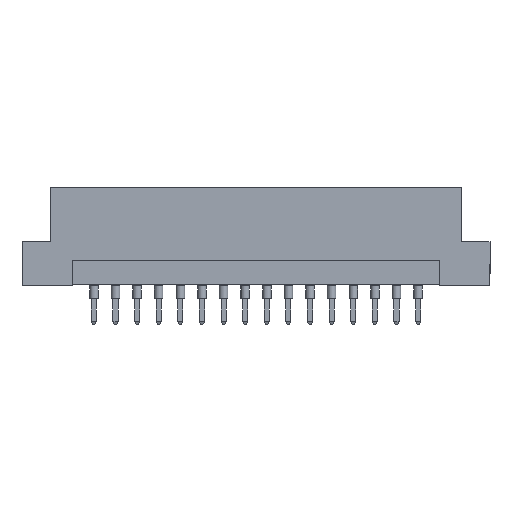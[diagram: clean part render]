
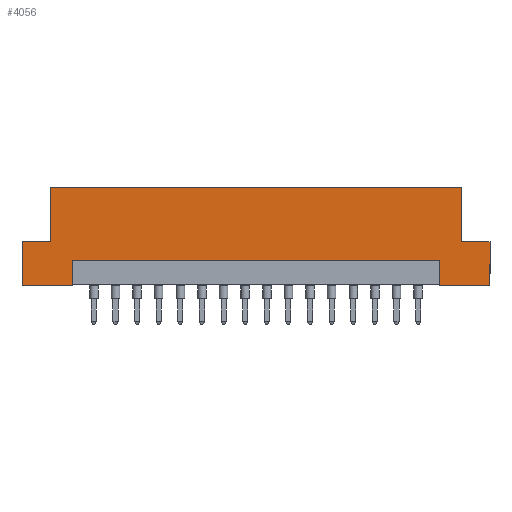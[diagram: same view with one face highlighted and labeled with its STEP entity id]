
A CAD part, front view. The second image highlights one B-rep face of the part: STEP entity #4056.
In plain terms, the highlighted planar face has unit normal (0, -1, 0).
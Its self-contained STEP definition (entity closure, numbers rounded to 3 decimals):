
#74 = EDGE_LOOP ( 'NONE', ( #4985, #642, #4675, #2474, #464, #729, #3918, #4071, #1507, #6756, #6027, #4657 ) ) ;
#327 = CARTESIAN_POINT ( 'NONE',  ( 21.6, -4.3, 0. ) ) ;
#408 = LINE ( 'NONE', #3615, #866 ) ;
#417 = CARTESIAN_POINT ( 'NONE',  ( -24.2, -4.3, 5.2 ) ) ;
#464 = ORIENTED_EDGE ( 'NONE', *, *, #3549, .F. ) ;
#532 = LINE ( 'NONE', #2778, #6791 ) ;
#642 = ORIENTED_EDGE ( 'NONE', *, *, #1631, .F. ) ;
#646 = VECTOR ( 'NONE', #2218, 1000. ) ;
#664 = CARTESIAN_POINT ( 'NONE',  ( -24.2, -4.3, 5.2 ) ) ;
#672 = CARTESIAN_POINT ( 'NONE',  ( 27.5, -4.3, 5.2 ) ) ;
#716 = LINE ( 'NONE', #3505, #4325 ) ;
#729 = ORIENTED_EDGE ( 'NONE', *, *, #5365, .T. ) ;
#774 = VERTEX_POINT ( 'NONE', #2461 ) ;
#866 = VECTOR ( 'NONE', #3646, 1000. ) ;
#1005 = CARTESIAN_POINT ( 'NONE',  ( -21.6, -4.3, 0.2 ) ) ;
#1081 = CARTESIAN_POINT ( 'NONE',  ( 24.2, -4.3, 5.2 ) ) ;
#1109 = DIRECTION ( 'NONE',  ( 0., 0., 1. ) ) ;
#1172 = VERTEX_POINT ( 'NONE', #5952 ) ;
#1237 = VECTOR ( 'NONE', #4430, 1000. ) ;
#1269 = EDGE_CURVE ( 'NONE', #4265, #2774, #5470, .T. ) ;
#1507 = ORIENTED_EDGE ( 'NONE', *, *, #3622, .F. ) ;
#1631 = EDGE_CURVE ( 'NONE', #4265, #3821, #3590, .T. ) ;
#1720 = EDGE_CURVE ( 'NONE', #774, #3821, #532, .T. ) ;
#1757 = CARTESIAN_POINT ( 'NONE',  ( -21.6, -4.3, 0. ) ) ;
#1794 = CARTESIAN_POINT ( 'NONE',  ( 24.2, -4.3, 5.2 ) ) ;
#1841 = VECTOR ( 'NONE', #5148, 1000. ) ;
#1904 = EDGE_CURVE ( 'NONE', #5167, #3651, #716, .T. ) ;
#2062 = DIRECTION ( 'NONE',  ( 0., 0., -1. ) ) ;
#2196 = LINE ( 'NONE', #1005, #6476 ) ;
#2218 = DIRECTION ( 'NONE',  ( 0., 0., 1. ) ) ;
#2461 = CARTESIAN_POINT ( 'NONE',  ( -21.6, -4.3, 3. ) ) ;
#2474 = ORIENTED_EDGE ( 'NONE', *, *, #5263, .F. ) ;
#2487 = DIRECTION ( 'NONE',  ( 0., 0., 1. ) ) ;
#2621 = CARTESIAN_POINT ( 'NONE',  ( 21.6, -4.3, 3. ) ) ;
#2671 = LINE ( 'NONE', #7101, #7029 ) ;
#2773 = EDGE_CURVE ( 'NONE', #5158, #5904, #5593, .T. ) ;
#2774 = VERTEX_POINT ( 'NONE', #5668 ) ;
#2778 = CARTESIAN_POINT ( 'NONE',  ( -21.6, -4.3, 3. ) ) ;
#2801 = PLANE ( 'NONE',  #5691 ) ;
#2835 = CARTESIAN_POINT ( 'NONE',  ( 27.5, -4.3, 11.6 ) ) ;
#3467 = LINE ( 'NONE', #5747, #1841 ) ;
#3503 = EDGE_CURVE ( 'NONE', #774, #3651, #2196, .T. ) ;
#3505 = CARTESIAN_POINT ( 'NONE',  ( 27.5, -4.3, 0. ) ) ;
#3549 = EDGE_CURVE ( 'NONE', #6982, #4794, #6265, .T. ) ;
#3590 = LINE ( 'NONE', #7066, #4130 ) ;
#3615 = CARTESIAN_POINT ( 'NONE',  ( 27.5, -4.3, 11.6 ) ) ;
#3617 = VECTOR ( 'NONE', #5949, 1000. ) ;
#3622 = EDGE_CURVE ( 'NONE', #4532, #5158, #3467, .T. ) ;
#3646 = DIRECTION ( 'NONE',  ( 1., 0., 0. ) ) ;
#3651 = VERTEX_POINT ( 'NONE', #1757 ) ;
#3821 = VERTEX_POINT ( 'NONE', #2621 ) ;
#3918 = ORIENTED_EDGE ( 'NONE', *, *, #5682, .F. ) ;
#3946 = LINE ( 'NONE', #1081, #6672 ) ;
#3962 = CARTESIAN_POINT ( 'NONE',  ( -27.5, -4.3, 5.2 ) ) ;
#4056 = ADVANCED_FACE ( 'NONE', ( #5628 ), #2801, .F. ) ;
#4071 = ORIENTED_EDGE ( 'NONE', *, *, #2773, .F. ) ;
#4130 = VECTOR ( 'NONE', #2487, 1000. ) ;
#4167 = VECTOR ( 'NONE', #4555, 1000. ) ;
#4265 = VERTEX_POINT ( 'NONE', #327 ) ;
#4325 = VECTOR ( 'NONE', #6272, 1000. ) ;
#4391 = DIRECTION ( 'NONE',  ( 1., 0., 0. ) ) ;
#4430 = DIRECTION ( 'NONE',  ( 1., 0., 0. ) ) ;
#4532 = VERTEX_POINT ( 'NONE', #3962 ) ;
#4555 = DIRECTION ( 'NONE',  ( 1., 0., 0. ) ) ;
#4657 = ORIENTED_EDGE ( 'NONE', *, *, #3503, .F. ) ;
#4675 = ORIENTED_EDGE ( 'NONE', *, *, #1269, .T. ) ;
#4755 = EDGE_CURVE ( 'NONE', #4532, #5167, #7070, .T. ) ;
#4794 = VERTEX_POINT ( 'NONE', #5432 ) ;
#4985 = ORIENTED_EDGE ( 'NONE', *, *, #1720, .T. ) ;
#5027 = DIRECTION ( 'NONE',  ( -1., 0., 0. ) ) ;
#5054 = CARTESIAN_POINT ( 'NONE',  ( 27.5, -4.3, 0. ) ) ;
#5104 = DIRECTION ( 'NONE',  ( 0., 1., 0. ) ) ;
#5148 = DIRECTION ( 'NONE',  ( 1., 0., 0. ) ) ;
#5158 = VERTEX_POINT ( 'NONE', #417 ) ;
#5167 = VERTEX_POINT ( 'NONE', #5941 ) ;
#5263 = EDGE_CURVE ( 'NONE', #4794, #2774, #2671, .T. ) ;
#5365 = EDGE_CURVE ( 'NONE', #6982, #1172, #3946, .T. ) ;
#5432 = CARTESIAN_POINT ( 'NONE',  ( 27.5, -4.3, 5.2 ) ) ;
#5465 = CARTESIAN_POINT ( 'NONE',  ( -27.5, -4.3, 11.6 ) ) ;
#5470 = LINE ( 'NONE', #5054, #1237 ) ;
#5562 = CARTESIAN_POINT ( 'NONE',  ( -24.2, -4.3, 11.6 ) ) ;
#5593 = LINE ( 'NONE', #664, #646 ) ;
#5628 = FACE_OUTER_BOUND ( 'NONE', #74, .T. ) ;
#5668 = CARTESIAN_POINT ( 'NONE',  ( 27.5, -4.3, 0. ) ) ;
#5682 = EDGE_CURVE ( 'NONE', #5904, #1172, #408, .T. ) ;
#5691 = AXIS2_PLACEMENT_3D ( 'NONE', #2835, #5104, #5027 ) ;
#5747 = CARTESIAN_POINT ( 'NONE',  ( -27.5, -4.3, 5.2 ) ) ;
#5904 = VERTEX_POINT ( 'NONE', #5562 ) ;
#5941 = CARTESIAN_POINT ( 'NONE',  ( -27.5, -4.3, 0. ) ) ;
#5949 = DIRECTION ( 'NONE',  ( 0., 0., -1. ) ) ;
#5952 = CARTESIAN_POINT ( 'NONE',  ( 24.2, -4.3, 11.6 ) ) ;
#6027 = ORIENTED_EDGE ( 'NONE', *, *, #1904, .T. ) ;
#6265 = LINE ( 'NONE', #672, #4167 ) ;
#6272 = DIRECTION ( 'NONE',  ( 1., 0., 0. ) ) ;
#6476 = VECTOR ( 'NONE', #7125, 1000. ) ;
#6672 = VECTOR ( 'NONE', #1109, 1000. ) ;
#6756 = ORIENTED_EDGE ( 'NONE', *, *, #4755, .T. ) ;
#6791 = VECTOR ( 'NONE', #4391, 1000. ) ;
#6982 = VERTEX_POINT ( 'NONE', #1794 ) ;
#7029 = VECTOR ( 'NONE', #2062, 1000. ) ;
#7066 = CARTESIAN_POINT ( 'NONE',  ( 21.6, -4.3, 0.2 ) ) ;
#7070 = LINE ( 'NONE', #5465, #3617 ) ;
#7101 = CARTESIAN_POINT ( 'NONE',  ( 27.5, -4.3, 11.6 ) ) ;
#7125 = DIRECTION ( 'NONE',  ( 0., 0., -1. ) ) ;
